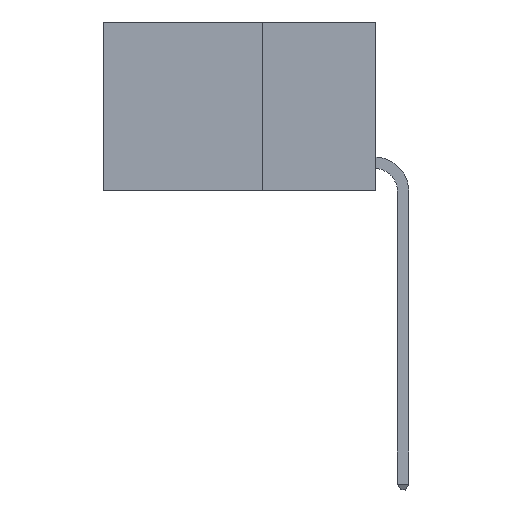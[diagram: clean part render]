
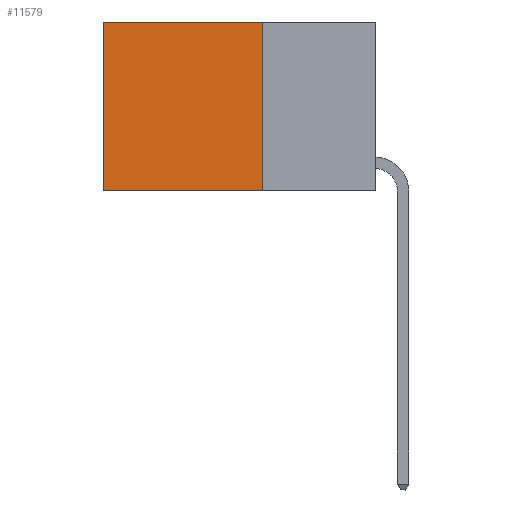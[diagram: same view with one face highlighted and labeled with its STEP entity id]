
A CAD part, left-side view. The second image highlights one B-rep face of the part: STEP entity #11579.
In plain terms, the highlighted planar face has unit normal (-1, 0, 0).
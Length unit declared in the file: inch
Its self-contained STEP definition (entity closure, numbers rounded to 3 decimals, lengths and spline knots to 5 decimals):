
#1266 = CARTESIAN_POINT ( 'NONE',  ( 0.2625, 0.25, 0. ) ) ;
#1408 = VERTEX_POINT ( 'NONE', #21446 ) ;
#1452 = VECTOR ( 'NONE', #20048, 39.37008 ) ;
#2538 = CARTESIAN_POINT ( 'NONE',  ( 0.2625, 0.25, 0. ) ) ;
#2976 = DIRECTION ( 'NONE',  ( 0., 0., -1. ) ) ;
#3292 = ORIENTED_EDGE ( 'NONE', *, *, #17355, .F. ) ;
#3473 = CARTESIAN_POINT ( 'NONE',  ( 0.2625, 0.25, -0.37 ) ) ;
#4954 = LINE ( 'NONE', #3473, #17922 ) ;
#5547 = CARTESIAN_POINT ( 'NONE',  ( 0.2625, 0.25, -0.37 ) ) ;
#5576 = VECTOR ( 'NONE', #9441, 39.37008 ) ;
#6795 = DIRECTION ( 'NONE',  ( 0., 0., -1. ) ) ;
#6822 = VERTEX_POINT ( 'NONE', #5547 ) ;
#8299 = LINE ( 'NONE', #2538, #5576 ) ;
#8406 = VECTOR ( 'NONE', #6795, 39.37008 ) ;
#8581 = CARTESIAN_POINT ( 'NONE',  ( 0.2625, 0.6, 0. ) ) ;
#9441 = DIRECTION ( 'NONE',  ( 0., 1., 0. ) ) ;
#10733 = VERTEX_POINT ( 'NONE', #16057 ) ;
#11579 = ADVANCED_FACE ( 'NONE', ( #16396 ), #21367, .F. ) ;
#11786 = CARTESIAN_POINT ( 'NONE',  ( 0.2625, 0.25, 0. ) ) ;
#11889 = ORIENTED_EDGE ( 'NONE', *, *, #16359, .F. ) ;
#12024 = DIRECTION ( 'NONE',  ( 0., 1., 0. ) ) ;
#12326 = EDGE_CURVE ( 'NONE', #10733, #14375, #17366, .T. ) ;
#13205 = DIRECTION ( 'NONE',  ( 1., 0., 0. ) ) ;
#13881 = EDGE_CURVE ( 'NONE', #1408, #10733, #8299, .T. ) ;
#14355 = AXIS2_PLACEMENT_3D ( 'NONE', #1266, #13205, #2976 ) ;
#14375 = VERTEX_POINT ( 'NONE', #15710 ) ;
#14467 = EDGE_LOOP ( 'NONE', ( #15850, #11889, #3292, #21152 ) ) ;
#15613 = LINE ( 'NONE', #11786, #1452 ) ;
#15710 = CARTESIAN_POINT ( 'NONE',  ( 0.2625, 0.6, -0.37 ) ) ;
#15850 = ORIENTED_EDGE ( 'NONE', *, *, #12326, .T. ) ;
#16057 = CARTESIAN_POINT ( 'NONE',  ( 0.2625, 0.6, 0. ) ) ;
#16359 = EDGE_CURVE ( 'NONE', #6822, #14375, #4954, .T. ) ;
#16396 = FACE_OUTER_BOUND ( 'NONE', #14467, .T. ) ;
#17355 = EDGE_CURVE ( 'NONE', #1408, #6822, #15613, .T. ) ;
#17366 = LINE ( 'NONE', #8581, #8406 ) ;
#17922 = VECTOR ( 'NONE', #12024, 39.37008 ) ;
#20048 = DIRECTION ( 'NONE',  ( 0., 0., -1. ) ) ;
#21152 = ORIENTED_EDGE ( 'NONE', *, *, #13881, .T. ) ;
#21367 = PLANE ( 'NONE',  #14355 ) ;
#21446 = CARTESIAN_POINT ( 'NONE',  ( 0.2625, 0.25, 0. ) ) ;
